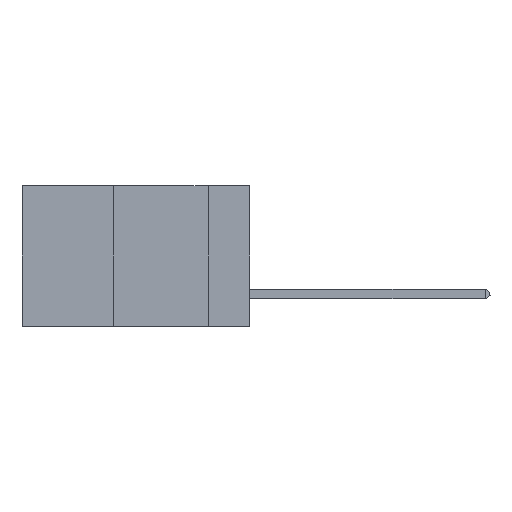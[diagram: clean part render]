
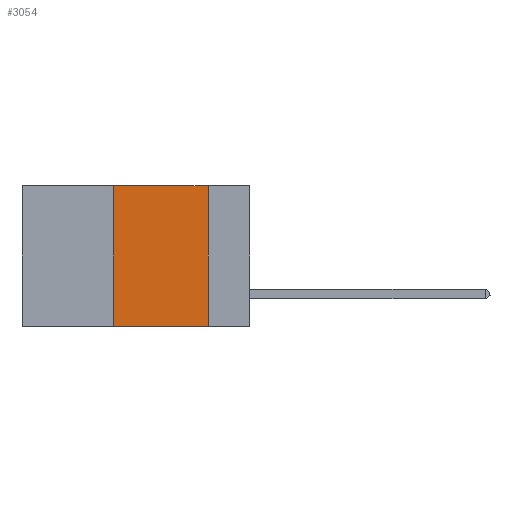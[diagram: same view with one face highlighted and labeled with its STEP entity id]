
A CAD part, left-side view. The second image highlights one B-rep face of the part: STEP entity #3054.
In plain terms, the highlighted planar face has unit normal (-1, 0, 0).
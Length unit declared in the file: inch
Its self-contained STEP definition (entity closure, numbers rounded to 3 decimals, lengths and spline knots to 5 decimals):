
#174 = VERTEX_POINT ( 'NONE', #10245 ) ;
#249 = EDGE_CURVE ( 'NONE', #3669, #709, #10466, .T. ) ;
#687 = VECTOR ( 'NONE', #10769, 39.37008 ) ;
#709 = VERTEX_POINT ( 'NONE', #10206 ) ;
#788 = DIRECTION ( 'NONE',  ( 0., 0., -1. ) ) ;
#1618 = EDGE_CURVE ( 'NONE', #4036, #709, #4343, .T. ) ;
#1708 = LINE ( 'NONE', #3272, #9751 ) ;
#1827 = ORIENTED_EDGE ( 'NONE', *, *, #8868, .F. ) ;
#1838 = DIRECTION ( 'NONE',  ( 0., 0., 1. ) ) ;
#2313 = DIRECTION ( 'NONE',  ( 0., 0., -1. ) ) ;
#2672 = CARTESIAN_POINT ( 'NONE',  ( 0., 0.6, -0.37 ) ) ;
#3054 = ADVANCED_FACE ( 'NONE', ( #9245 ), #3196, .F. ) ;
#3164 = EDGE_CURVE ( 'NONE', #174, #3669, #1708, .T. ) ;
#3196 = PLANE ( 'NONE',  #9795 ) ;
#3272 = CARTESIAN_POINT ( 'NONE',  ( 0., 0.6, 0. ) ) ;
#3291 = EDGE_LOOP ( 'NONE', ( #8524, #10169, #1827, #7378 ) ) ;
#3668 = VECTOR ( 'NONE', #1838, 39.37008 ) ;
#3669 = VERTEX_POINT ( 'NONE', #8310 ) ;
#4036 = VERTEX_POINT ( 'NONE', #8124 ) ;
#4343 = LINE ( 'NONE', #2672, #687 ) ;
#4581 = CARTESIAN_POINT ( 'NONE',  ( 0., 0.11, 0. ) ) ;
#4731 = DIRECTION ( 'NONE',  ( 1., 0., 0. ) ) ;
#7378 = ORIENTED_EDGE ( 'NONE', *, *, #1618, .T. ) ;
#8124 = CARTESIAN_POINT ( 'NONE',  ( 0., 0.36, -0.37 ) ) ;
#8293 = DIRECTION ( 'NONE',  ( 0., -1., 0. ) ) ;
#8310 = CARTESIAN_POINT ( 'NONE',  ( 0., 0.11, 0. ) ) ;
#8524 = ORIENTED_EDGE ( 'NONE', *, *, #249, .F. ) ;
#8853 = CARTESIAN_POINT ( 'NONE',  ( 0., 0.6, 0. ) ) ;
#8868 = EDGE_CURVE ( 'NONE', #4036, #174, #10530, .T. ) ;
#8901 = VECTOR ( 'NONE', #2313, 39.37008 ) ;
#9245 = FACE_OUTER_BOUND ( 'NONE', #3291, .T. ) ;
#9751 = VECTOR ( 'NONE', #8293, 39.37008 ) ;
#9795 = AXIS2_PLACEMENT_3D ( 'NONE', #8853, #4731, #788 ) ;
#10169 = ORIENTED_EDGE ( 'NONE', *, *, #3164, .F. ) ;
#10189 = CARTESIAN_POINT ( 'NONE',  ( 0., 0.36, 0. ) ) ;
#10206 = CARTESIAN_POINT ( 'NONE',  ( 0., 0.11, -0.37 ) ) ;
#10245 = CARTESIAN_POINT ( 'NONE',  ( 0., 0.36, 0. ) ) ;
#10466 = LINE ( 'NONE', #4581, #8901 ) ;
#10530 = LINE ( 'NONE', #10189, #3668 ) ;
#10769 = DIRECTION ( 'NONE',  ( 0., -1., 0. ) ) ;
